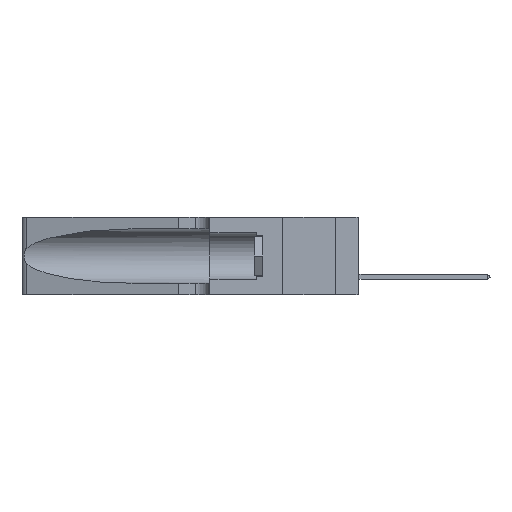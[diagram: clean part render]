
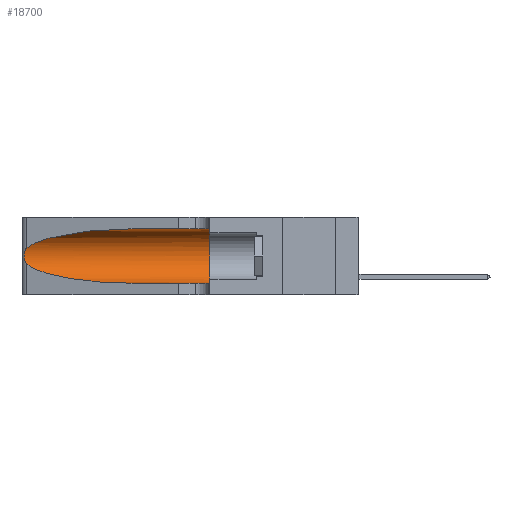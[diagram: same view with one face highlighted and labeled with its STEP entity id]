
A CAD part, left-side view. The second image highlights one B-rep face of the part: STEP entity #18700.
In plain terms, the highlighted cylindrical face has radius 3.308 mm (diameter 6.617 mm), a partial arc.
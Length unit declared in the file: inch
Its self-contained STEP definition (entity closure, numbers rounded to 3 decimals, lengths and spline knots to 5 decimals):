
#24 = LINE ( 'NONE', #8352, #18778 ) ;
#691 = CARTESIAN_POINT ( 'NONE',  ( 0.25487, 1.22718, 0.22369 ) ) ;
#772 = CARTESIAN_POINT ( 'NONE',  ( 0.25487, 1.22718, 0.14631 ) ) ;
#778 = CARTESIAN_POINT ( 'NONE',  ( 0.1305, 1.61858, 0.31525 ) ) ;
#969 = DIRECTION ( 'NONE',  ( 0., 0., -1. ) ) ;
#1097 = EDGE_CURVE ( 'NONE', #18998, #13052, #24, .T. ) ;
#1373 = CARTESIAN_POINT ( 'NONE',  ( 0.2373, 1.15595, 0.28018 ) ) ;
#2083 = DIRECTION ( 'NONE',  ( 0., 1., 0. ) ) ;
#2108 = FACE_OUTER_BOUND ( 'NONE', #12626, .T. ) ;
#2161 = AXIS2_PLACEMENT_3D ( 'NONE', #2431, #11203, #969 ) ;
#2431 = CARTESIAN_POINT ( 'NONE',  ( 0.1305, 1.61858, 0.185 ) ) ;
#3394 = CARTESIAN_POINT ( 'NONE',  ( 0.25487, 1.22718, 0.22369 ) ) ;
#4340 =( BOUNDED_CURVE ( )  B_SPLINE_CURVE ( 3, ( #14642, #9390, #14716, #10522 ),
 .UNSPECIFIED., .F., .F. ) 
 B_SPLINE_CURVE_WITH_KNOTS ( ( 4, 4 ),
 ( 3.44316, 4.71239 ),
 .UNSPECIFIED. ) 
 CURVE ( )  GEOMETRIC_REPRESENTATION_ITEM ( )  RATIONAL_B_SPLINE_CURVE ( ( 1., 0.87, 0.87, 1. ) ) 
 REPRESENTATION_ITEM ( '' )  );
#4341 = CARTESIAN_POINT ( 'NONE',  ( 0.25856, 1.23593, 0.16098 ) ) ;
#4415 = CARTESIAN_POINT ( 'NONE',  ( 0.25639, 1.23184, 0.21858 ) ) ;
#4918 = VERTEX_POINT ( 'NONE', #6202 ) ;
#5011 = CARTESIAN_POINT ( 'NONE',  ( 0.18966, 0.96281, 0.31525 ) ) ;
#5469 = DIRECTION ( 'NONE',  ( 0., 0., 1. ) ) ;
#6082 = CARTESIAN_POINT ( 'NONE',  ( 0.25555, 1.22994, 0.2215 ) ) ;
#6202 = CARTESIAN_POINT ( 'NONE',  ( 0.1305, 0.35, 0.31525 ) ) ;
#6239 = CARTESIAN_POINT ( 'NONE',  ( 0.26018, 1.23835, 0.19895 ) ) ;
#6898 = VECTOR ( 'NONE', #20547, 39.37008 ) ;
#7275 = VERTEX_POINT ( 'NONE', #21611 ) ;
#7381 = EDGE_CURVE ( 'NONE', #4918, #13052, #10948, .T. ) ;
#7886 = CARTESIAN_POINT ( 'NONE',  ( 0.25854, 1.2359, 0.20912 ) ) ;
#8352 = CARTESIAN_POINT ( 'NONE',  ( 0.1305, 1.61858, 0.05475 ) ) ;
#8395 = CARTESIAN_POINT ( 'NONE',  ( 0.1305, 0.72297, 0.31525 ) ) ;
#8936 = CARTESIAN_POINT ( 'NONE',  ( 0.1305, 0.35, 0.185 ) ) ;
#9390 = CARTESIAN_POINT ( 'NONE',  ( 0.2373, 1.15595, 0.08982 ) ) ;
#9558 = CARTESIAN_POINT ( 'NONE',  ( 0.26017, 1.23833, 0.17102 ) ) ;
#9716 = CARTESIAN_POINT ( 'NONE',  ( 0.25555, 1.22993, 0.14849 ) ) ;
#10522 = CARTESIAN_POINT ( 'NONE',  ( 0.1305, 0.72297, 0.05475 ) ) ;
#10814 = B_SPLINE_CURVE_WITH_KNOTS ( 'NONE', 3,
 ( #691, #6082, #4415, #20151, #7886, #6239, #11171, #20223, #9558, #4341, #15062, #13110, #9716, #772 ),
 .UNSPECIFIED., .F., .F.,
 ( 4, 2, 2, 2, 2, 2, 4 ),
 ( 0., 0.00027, 0.00053, 0.00107, 0.0016, 0.00187, 0.00214 ),
 .UNSPECIFIED. ) ;
#10948 = CIRCLE ( 'NONE', #14402, 0.13025 ) ;
#11171 = CARTESIAN_POINT ( 'NONE',  ( 0.26075, 1.23896, 0.19203 ) ) ;
#11203 = DIRECTION ( 'NONE',  ( 0., -1., 0. ) ) ;
#11225 = EDGE_CURVE ( 'NONE', #15497, #22114, #14227, .T. ) ;
#12626 = EDGE_LOOP ( 'NONE', ( #20229, #14993, #22434, #13299, #17449, #18914 ) ) ;
#13052 = VERTEX_POINT ( 'NONE', #18456 ) ;
#13110 = CARTESIAN_POINT ( 'NONE',  ( 0.25639, 1.23186, 0.15144 ) ) ;
#13299 = ORIENTED_EDGE ( 'NONE', *, *, #1097, .T. ) ;
#13696 = CYLINDRICAL_SURFACE ( 'NONE', #2161, 0.13025 ) ;
#14227 =( BOUNDED_CURVE ( )  B_SPLINE_CURVE ( 3, ( #8395, #5011, #1373, #3394 ),
 .UNSPECIFIED., .F., .T. ) 
 B_SPLINE_CURVE_WITH_KNOTS ( ( 4, 4 ),
 ( 1.5708, 2.84003 ),
 .UNSPECIFIED. ) 
 CURVE ( )  GEOMETRIC_REPRESENTATION_ITEM ( )  RATIONAL_B_SPLINE_CURVE ( ( 1., 0.87, 0.87, 1. ) ) 
 REPRESENTATION_ITEM ( '' )  );
#14402 = AXIS2_PLACEMENT_3D ( 'NONE', #8936, #2083, #5469 ) ;
#14642 = CARTESIAN_POINT ( 'NONE',  ( 0.25487, 1.22718, 0.14631 ) ) ;
#14716 = CARTESIAN_POINT ( 'NONE',  ( 0.18966, 0.96281, 0.05475 ) ) ;
#14993 = ORIENTED_EDGE ( 'NONE', *, *, #20124, .T. ) ;
#15062 = CARTESIAN_POINT ( 'NONE',  ( 0.25789, 1.23486, 0.15765 ) ) ;
#15497 = VERTEX_POINT ( 'NONE', #19090 ) ;
#16162 = CARTESIAN_POINT ( 'NONE',  ( 0.1305, 0.72297, 0.05475 ) ) ;
#16632 = EDGE_CURVE ( 'NONE', #15497, #4918, #19787, .T. ) ;
#17449 = ORIENTED_EDGE ( 'NONE', *, *, #7381, .F. ) ;
#18456 = CARTESIAN_POINT ( 'NONE',  ( 0.1305, 0.35, 0.05475 ) ) ;
#18700 = ADVANCED_FACE ( 'NONE', ( #2108 ), #13696, .F. ) ;
#18778 = VECTOR ( 'NONE', #18800, 39.37008 ) ;
#18800 = DIRECTION ( 'NONE',  ( 0., -1., 0. ) ) ;
#18914 = ORIENTED_EDGE ( 'NONE', *, *, #16632, .F. ) ;
#18998 = VERTEX_POINT ( 'NONE', #16162 ) ;
#19090 = CARTESIAN_POINT ( 'NONE',  ( 0.1305, 0.72297, 0.31525 ) ) ;
#19787 = LINE ( 'NONE', #778, #6898 ) ;
#19794 = EDGE_CURVE ( 'NONE', #7275, #18998, #4340, .T. ) ;
#19916 = CARTESIAN_POINT ( 'NONE',  ( 0.25487, 1.22718, 0.22369 ) ) ;
#20124 = EDGE_CURVE ( 'NONE', #22114, #7275, #10814, .T. ) ;
#20151 = CARTESIAN_POINT ( 'NONE',  ( 0.25787, 1.23484, 0.2124 ) ) ;
#20223 = CARTESIAN_POINT ( 'NONE',  ( 0.26075, 1.23896, 0.178 ) ) ;
#20229 = ORIENTED_EDGE ( 'NONE', *, *, #11225, .T. ) ;
#20547 = DIRECTION ( 'NONE',  ( 0., -1., 0. ) ) ;
#21611 = CARTESIAN_POINT ( 'NONE',  ( 0.25487, 1.22718, 0.14631 ) ) ;
#22114 = VERTEX_POINT ( 'NONE', #19916 ) ;
#22434 = ORIENTED_EDGE ( 'NONE', *, *, #19794, .T. ) ;
